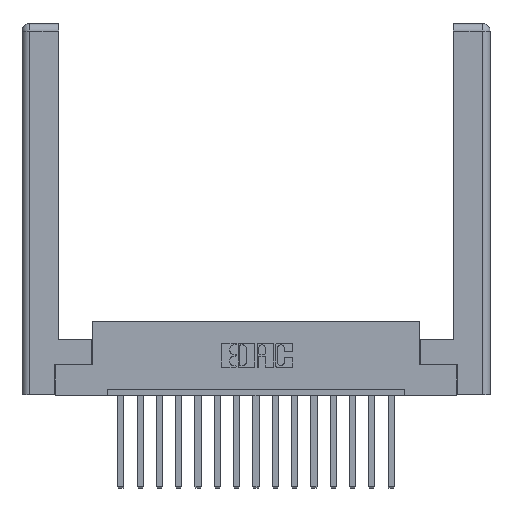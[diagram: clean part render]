
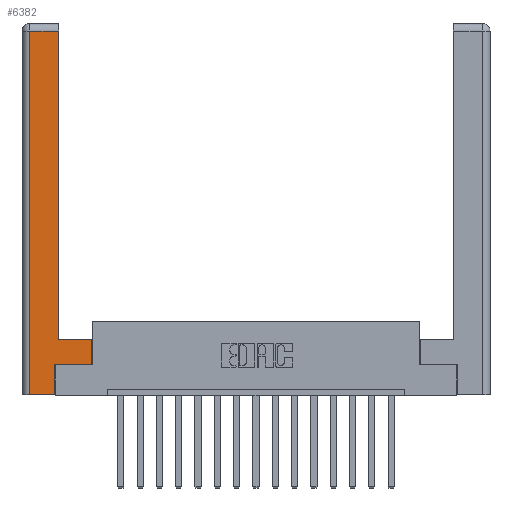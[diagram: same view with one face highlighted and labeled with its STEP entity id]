
A CAD part, top view. The second image highlights one B-rep face of the part: STEP entity #6382.
In plain terms, the highlighted planar face has unit normal (0, 0, 1).
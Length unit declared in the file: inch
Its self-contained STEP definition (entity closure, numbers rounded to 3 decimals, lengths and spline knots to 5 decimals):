
#363 = ORIENTED_EDGE ( 'NONE', *, *, #4862, .T. ) ;
#660 = FACE_OUTER_BOUND ( 'NONE', #8148, .T. ) ;
#844 = VERTEX_POINT ( 'NONE', #1461 ) ;
#872 = VERTEX_POINT ( 'NONE', #4168 ) ;
#1030 = VERTEX_POINT ( 'NONE', #2136 ) ;
#1225 = EDGE_CURVE ( 'NONE', #5552, #5597, #3115, .T. ) ;
#1461 = CARTESIAN_POINT ( 'NONE',  ( 0.0615, 0., 0. ) ) ;
#1606 = ORIENTED_EDGE ( 'NONE', *, *, #1225, .T. ) ;
#1634 = EDGE_CURVE ( 'NONE', #5597, #10248, #14472, .T. ) ;
#1673 = CARTESIAN_POINT ( 'NONE',  ( 0.0615, 0., 0. ) ) ;
#1810 = CARTESIAN_POINT ( 'NONE',  ( 0.565, 0.45, 0. ) ) ;
#1999 = CARTESIAN_POINT ( 'NONE',  ( 0.565, 0.245, 0. ) ) ;
#2136 = CARTESIAN_POINT ( 'NONE',  ( 0.295, 0.45, 0. ) ) ;
#2203 = ORIENTED_EDGE ( 'NONE', *, *, #9417, .T. ) ;
#2450 = AXIS2_PLACEMENT_3D ( 'NONE', #13827, #5946, #15171 ) ;
#2517 = LINE ( 'NONE', #13712, #4999 ) ;
#2638 = ORIENTED_EDGE ( 'NONE', *, *, #14437, .T. ) ;
#2740 = VECTOR ( 'NONE', #7801, 39.37008 ) ;
#2788 = CARTESIAN_POINT ( 'NONE',  ( 0.265, 0., 0. ) ) ;
#3115 = LINE ( 'NONE', #9903, #10575 ) ;
#3136 = LINE ( 'NONE', #16925, #2740 ) ;
#3166 = VERTEX_POINT ( 'NONE', #5443 ) ;
#3426 = PLANE ( 'NONE',  #2450 ) ;
#3513 = EDGE_CURVE ( 'NONE', #3166, #844, #13947, .T. ) ;
#3661 = DIRECTION ( 'NONE',  ( -1., 0., 0. ) ) ;
#3844 = VECTOR ( 'NONE', #4267, 39.37008 ) ;
#4168 = CARTESIAN_POINT ( 'NONE',  ( 0.265, 0., 0. ) ) ;
#4267 = DIRECTION ( 'NONE',  ( 0., -1., 0. ) ) ;
#4517 = DIRECTION ( 'NONE',  ( 1., 0., 0. ) ) ;
#4546 = CARTESIAN_POINT ( 'NONE',  ( 0.295, 2.94, 0. ) ) ;
#4862 = EDGE_CURVE ( 'NONE', #10248, #1030, #7982, .T. ) ;
#4999 = VECTOR ( 'NONE', #16470, 39.37008 ) ;
#5063 = CARTESIAN_POINT ( 'NONE',  ( 0.0615, 2.94, 0. ) ) ;
#5443 = CARTESIAN_POINT ( 'NONE',  ( 0.0615, 2.94, 0. ) ) ;
#5552 = VERTEX_POINT ( 'NONE', #11187 ) ;
#5597 = VERTEX_POINT ( 'NONE', #1999 ) ;
#5794 = DIRECTION ( 'NONE',  ( 1., 0., 0. ) ) ;
#5946 = DIRECTION ( 'NONE',  ( 0., 0., -1. ) ) ;
#5948 = DIRECTION ( 'NONE',  ( -1., 0., 0. ) ) ;
#6382 = ADVANCED_FACE ( 'NONE', ( #660 ), #3426, .F. ) ;
#6405 = VERTEX_POINT ( 'NONE', #4546 ) ;
#6431 = EDGE_CURVE ( 'NONE', #1030, #6405, #2517, .T. ) ;
#6704 = EDGE_CURVE ( 'NONE', #872, #5552, #3136, .T. ) ;
#6821 = VECTOR ( 'NONE', #3661, 39.37008 ) ;
#7510 = ORIENTED_EDGE ( 'NONE', *, *, #3513, .T. ) ;
#7801 = DIRECTION ( 'NONE',  ( 0., 1., 0. ) ) ;
#7834 = LINE ( 'NONE', #5063, #6821 ) ;
#7982 = LINE ( 'NONE', #8782, #13505 ) ;
#8148 = EDGE_LOOP ( 'NONE', ( #10369, #2638, #7510, #2203, #10208, #1606, #15489, #363 ) ) ;
#8485 = VECTOR ( 'NONE', #10235, 39.37008 ) ;
#8782 = CARTESIAN_POINT ( 'NONE',  ( 0.295, 0.45, 0. ) ) ;
#9029 = LINE ( 'NONE', #2788, #16837 ) ;
#9417 = EDGE_CURVE ( 'NONE', #844, #872, #9029, .T. ) ;
#9903 = CARTESIAN_POINT ( 'NONE',  ( 0.565, 0.245, 0. ) ) ;
#10063 = CARTESIAN_POINT ( 'NONE',  ( 0.565, 0.45, 0. ) ) ;
#10208 = ORIENTED_EDGE ( 'NONE', *, *, #6704, .T. ) ;
#10235 = DIRECTION ( 'NONE',  ( 0., 1., 0. ) ) ;
#10248 = VERTEX_POINT ( 'NONE', #1810 ) ;
#10369 = ORIENTED_EDGE ( 'NONE', *, *, #6431, .T. ) ;
#10575 = VECTOR ( 'NONE', #4517, 39.37008 ) ;
#11187 = CARTESIAN_POINT ( 'NONE',  ( 0.265, 0.245, 0. ) ) ;
#13505 = VECTOR ( 'NONE', #5948, 39.37008 ) ;
#13712 = CARTESIAN_POINT ( 'NONE',  ( 0.295, 3., 0. ) ) ;
#13827 = CARTESIAN_POINT ( 'NONE',  ( 0., 0., 0. ) ) ;
#13947 = LINE ( 'NONE', #1673, #3844 ) ;
#14437 = EDGE_CURVE ( 'NONE', #6405, #3166, #7834, .T. ) ;
#14472 = LINE ( 'NONE', #10063, #8485 ) ;
#15171 = DIRECTION ( 'NONE',  ( -1., 0., 0. ) ) ;
#15489 = ORIENTED_EDGE ( 'NONE', *, *, #1634, .T. ) ;
#16470 = DIRECTION ( 'NONE',  ( 0., 1., 0. ) ) ;
#16837 = VECTOR ( 'NONE', #5794, 39.37008 ) ;
#16925 = CARTESIAN_POINT ( 'NONE',  ( 0.265, 0.245, 0. ) ) ;
